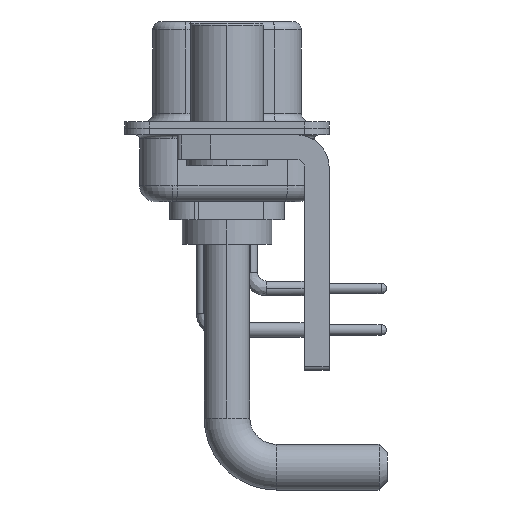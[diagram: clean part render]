
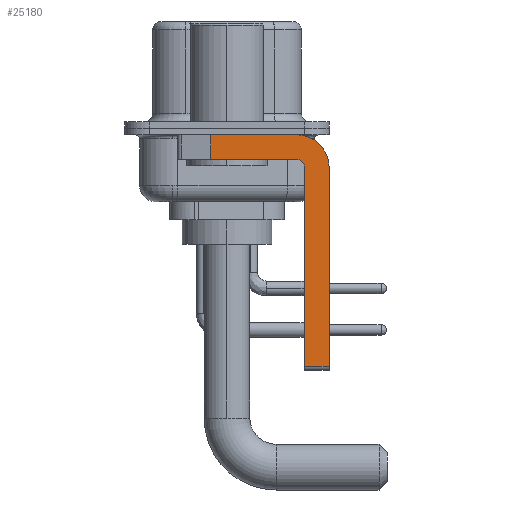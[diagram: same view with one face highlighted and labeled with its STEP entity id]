
A CAD part, left-side view. The second image highlights one B-rep face of the part: STEP entity #25180.
In plain terms, the highlighted planar face has unit normal (-1, 0, 0).
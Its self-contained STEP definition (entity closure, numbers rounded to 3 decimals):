
#318 = EDGE_CURVE ( 'NONE', #20416, #655, #18089, .T. ) ;
#655 = VERTEX_POINT ( 'NONE', #17210 ) ;
#1602 = VECTOR ( 'NONE', #7340, 1000. ) ;
#2614 = DIRECTION ( 'NONE',  ( 1., 0., 0. ) ) ;
#3174 = CARTESIAN_POINT ( 'NONE',  ( -2.9, 0.978, -1.9 ) ) ;
#3258 = EDGE_CURVE ( 'NONE', #29428, #20416, #17217, .T. ) ;
#3303 = ORIENTED_EDGE ( 'NONE', *, *, #3258, .F. ) ;
#4198 = CARTESIAN_POINT ( 'NONE',  ( -2.9, -4.75, -14.55 ) ) ;
#4801 = VERTEX_POINT ( 'NONE', #4925 ) ;
#4804 = PLANE ( 'NONE',  #15375 ) ;
#4925 = CARTESIAN_POINT ( 'NONE',  ( -2.9, -4.25, -0.4 ) ) ;
#5010 = VERTEX_POINT ( 'NONE', #21037 ) ;
#5456 = CARTESIAN_POINT ( 'NONE',  ( -2.9, -4.75, -14.8 ) ) ;
#6195 = VERTEX_POINT ( 'NONE', #19831 ) ;
#6611 = ORIENTED_EDGE ( 'NONE', *, *, #25634, .F. ) ;
#6626 = CARTESIAN_POINT ( 'NONE',  ( -2.9, 0.978, -1.9 ) ) ;
#7340 = DIRECTION ( 'NONE',  ( 0., 0., 1. ) ) ;
#7451 = DIRECTION ( 'NONE',  ( 0., -1., 0. ) ) ;
#7477 = ORIENTED_EDGE ( 'NONE', *, *, #26158, .T. ) ;
#8678 = ORIENTED_EDGE ( 'NONE', *, *, #22019, .F. ) ;
#8712 = CARTESIAN_POINT ( 'NONE',  ( -2.9, -4.25, -2.4 ) ) ;
#8861 = AXIS2_PLACEMENT_3D ( 'NONE', #26745, #10236, #27205 ) ;
#9623 = VECTOR ( 'NONE', #21720, 1000. ) ;
#9972 = LINE ( 'NONE', #21917, #16753 ) ;
#10236 = DIRECTION ( 'NONE',  ( 1., 0., 0. ) ) ;
#10794 = CARTESIAN_POINT ( 'NONE',  ( -2.9, -4.75, -2.4 ) ) ;
#10843 = VERTEX_POINT ( 'NONE', #14904 ) ;
#11417 = VECTOR ( 'NONE', #22294, 1000. ) ;
#12158 = DIRECTION ( 'NONE',  ( 0., 0., -1. ) ) ;
#12712 = LINE ( 'NONE', #3174, #11417 ) ;
#13730 = DIRECTION ( 'NONE',  ( -1., 0., 0. ) ) ;
#14062 = LINE ( 'NONE', #20996, #27276 ) ;
#14351 = CARTESIAN_POINT ( 'NONE',  ( -2.9, -4.25, -2.4 ) ) ;
#14481 = CARTESIAN_POINT ( 'NONE',  ( -2.9, -4.25, -1.9 ) ) ;
#14904 = CARTESIAN_POINT ( 'NONE',  ( -2.9, -6.25, -14.55 ) ) ;
#15375 = AXIS2_PLACEMENT_3D ( 'NONE', #14351, #2614, #12158 ) ;
#15545 = ORIENTED_EDGE ( 'NONE', *, *, #16467, .F. ) ;
#16398 = CIRCLE ( 'NONE', #8861, 2. ) ;
#16467 = EDGE_CURVE ( 'NONE', #655, #19728, #19683, .T. ) ;
#16753 = VECTOR ( 'NONE', #26806, 1000. ) ;
#16760 = DIRECTION ( 'NONE',  ( 0., 0., -1. ) ) ;
#17210 = CARTESIAN_POINT ( 'NONE',  ( -2.9, -4.25, -1.9 ) ) ;
#17217 = LINE ( 'NONE', #5456, #1602 ) ;
#18089 = CIRCLE ( 'NONE', #19086, 0.5 ) ;
#19086 = AXIS2_PLACEMENT_3D ( 'NONE', #8712, #13730, #20817 ) ;
#19683 = LINE ( 'NONE', #14481, #9623 ) ;
#19728 = VERTEX_POINT ( 'NONE', #6626 ) ;
#19831 = CARTESIAN_POINT ( 'NONE',  ( -2.9, -6.25, -2.4 ) ) ;
#20416 = VERTEX_POINT ( 'NONE', #10794 ) ;
#20457 = EDGE_LOOP ( 'NONE', ( #21060, #7477, #15545, #26001, #3303, #26963, #8678, #6611 ) ) ;
#20817 = DIRECTION ( 'NONE',  ( 0., 0., 1. ) ) ;
#20996 = CARTESIAN_POINT ( 'NONE',  ( -2.9, -6.25, -2.4 ) ) ;
#21037 = CARTESIAN_POINT ( 'NONE',  ( -2.9, 0.978, -0.4 ) ) ;
#21060 = ORIENTED_EDGE ( 'NONE', *, *, #22720, .F. ) ;
#21720 = DIRECTION ( 'NONE',  ( 0., 1., 0. ) ) ;
#21740 = FACE_OUTER_BOUND ( 'NONE', #20457, .T. ) ;
#21917 = CARTESIAN_POINT ( 'NONE',  ( -2.9, -4.25, -14.55 ) ) ;
#22019 = EDGE_CURVE ( 'NONE', #6195, #10843, #14062, .T. ) ;
#22293 = VECTOR ( 'NONE', #7451, 1000. ) ;
#22294 = DIRECTION ( 'NONE',  ( 0., 0., -1. ) ) ;
#22330 = EDGE_CURVE ( 'NONE', #29428, #10843, #9972, .T. ) ;
#22720 = EDGE_CURVE ( 'NONE', #5010, #4801, #24403, .T. ) ;
#24403 = LINE ( 'NONE', #29600, #22293 ) ;
#25180 = ADVANCED_FACE ( 'NONE', ( #21740 ), #4804, .F. ) ;
#25634 = EDGE_CURVE ( 'NONE', #4801, #6195, #16398, .T. ) ;
#26001 = ORIENTED_EDGE ( 'NONE', *, *, #318, .F. ) ;
#26158 = EDGE_CURVE ( 'NONE', #5010, #19728, #12712, .T. ) ;
#26745 = CARTESIAN_POINT ( 'NONE',  ( -2.9, -4.25, -2.4 ) ) ;
#26806 = DIRECTION ( 'NONE',  ( 0., -1., 0. ) ) ;
#26963 = ORIENTED_EDGE ( 'NONE', *, *, #22330, .T. ) ;
#27205 = DIRECTION ( 'NONE',  ( 0., 0., -1. ) ) ;
#27276 = VECTOR ( 'NONE', #16760, 1000. ) ;
#29428 = VERTEX_POINT ( 'NONE', #4198 ) ;
#29600 = CARTESIAN_POINT ( 'NONE',  ( -2.9, 3., -0.4 ) ) ;
